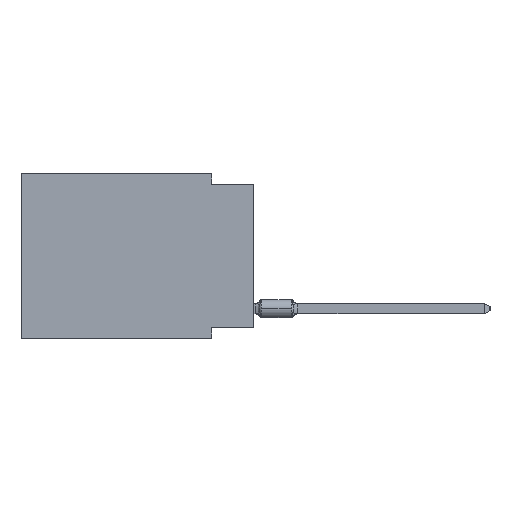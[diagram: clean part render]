
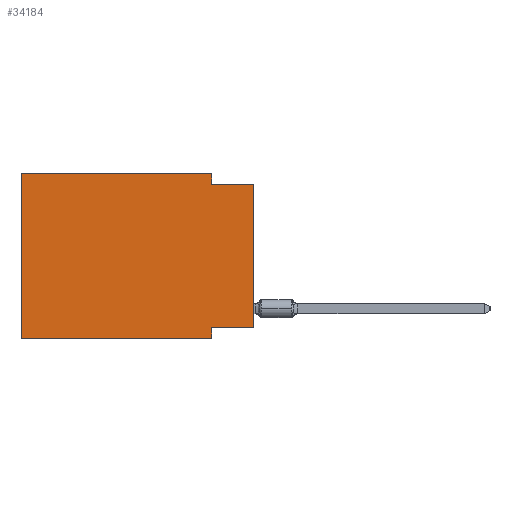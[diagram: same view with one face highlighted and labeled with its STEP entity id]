
A CAD part, left-side view. The second image highlights one B-rep face of the part: STEP entity #34184.
In plain terms, the highlighted planar face has unit normal (-1, 0, 0).
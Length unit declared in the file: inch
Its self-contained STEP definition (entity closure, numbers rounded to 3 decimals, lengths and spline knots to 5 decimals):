
#429 = VECTOR ( 'NONE', #16689, 39.37008 ) ;
#627 = EDGE_CURVE ( 'NONE', #7368, #34009, #24942, .T. ) ;
#677 = VERTEX_POINT ( 'NONE', #8604 ) ;
#1767 = PLANE ( 'NONE',  #8205 ) ;
#2180 = DIRECTION ( 'NONE',  ( 0., 0., 1. ) ) ;
#2861 = DIRECTION ( 'NONE',  ( 0., 0., -1. ) ) ;
#3881 = CARTESIAN_POINT ( 'NONE',  ( 0., 0.55, 0. ) ) ;
#3949 = ORIENTED_EDGE ( 'NONE', *, *, #627, .F. ) ;
#4445 = DIRECTION ( 'NONE',  ( 0., 0., -1. ) ) ;
#4621 = EDGE_LOOP ( 'NONE', ( #34359, #3949, #6401, #26085, #5821, #31547, #30589, #5751 ) ) ;
#4941 = CARTESIAN_POINT ( 'NONE',  ( 0., 0.55, -0.39 ) ) ;
#5213 = VECTOR ( 'NONE', #2861, 39.37008 ) ;
#5252 = VERTEX_POINT ( 'NONE', #3881 ) ;
#5419 = CARTESIAN_POINT ( 'NONE',  ( 0., 0.1, 0. ) ) ;
#5643 = CARTESIAN_POINT ( 'NONE',  ( 0., 0., -0.025 ) ) ;
#5751 = ORIENTED_EDGE ( 'NONE', *, *, #22914, .F. ) ;
#5821 = ORIENTED_EDGE ( 'NONE', *, *, #23498, .F. ) ;
#6401 = ORIENTED_EDGE ( 'NONE', *, *, #6893, .F. ) ;
#6648 = CARTESIAN_POINT ( 'NONE',  ( 0., 0., -0.365 ) ) ;
#6893 = EDGE_CURVE ( 'NONE', #10375, #7368, #22031, .T. ) ;
#7368 = VERTEX_POINT ( 'NONE', #21632 ) ;
#7460 = LINE ( 'NONE', #28712, #13369 ) ;
#7927 = VECTOR ( 'NONE', #4445, 39.37008 ) ;
#8205 = AXIS2_PLACEMENT_3D ( 'NONE', #25989, #28633, #14948 ) ;
#8383 = LINE ( 'NONE', #21924, #10924 ) ;
#8421 = CARTESIAN_POINT ( 'NONE',  ( 0., 0., -0.025 ) ) ;
#8604 = CARTESIAN_POINT ( 'NONE',  ( 0., 0.1, -0.365 ) ) ;
#9453 = LINE ( 'NONE', #6648, #29624 ) ;
#9874 = DIRECTION ( 'NONE',  ( 0., 0., 1. ) ) ;
#10375 = VERTEX_POINT ( 'NONE', #5419 ) ;
#10924 = VECTOR ( 'NONE', #32270, 39.37008 ) ;
#11708 = EDGE_CURVE ( 'NONE', #5252, #10375, #8383, .T. ) ;
#13369 = VECTOR ( 'NONE', #2180, 39.37008 ) ;
#14948 = DIRECTION ( 'NONE',  ( 0., 0., -1. ) ) ;
#15497 = LINE ( 'NONE', #25687, #28084 ) ;
#15819 = VECTOR ( 'NONE', #31308, 39.37008 ) ;
#16689 = DIRECTION ( 'NONE',  ( 0., -1., 0. ) ) ;
#16751 = CARTESIAN_POINT ( 'NONE',  ( 0., 0.1, 0. ) ) ;
#20670 = EDGE_CURVE ( 'NONE', #31798, #34009, #15497, .T. ) ;
#21632 = CARTESIAN_POINT ( 'NONE',  ( 0., 0.1, -0.025 ) ) ;
#21763 = CARTESIAN_POINT ( 'NONE',  ( 0., 0., -0.365 ) ) ;
#21790 = EDGE_CURVE ( 'NONE', #21901, #29143, #34292, .T. ) ;
#21901 = VERTEX_POINT ( 'NONE', #33774 ) ;
#21924 = CARTESIAN_POINT ( 'NONE',  ( 0., 0.55, 0. ) ) ;
#22031 = LINE ( 'NONE', #16751, #5213 ) ;
#22914 = EDGE_CURVE ( 'NONE', #31798, #677, #9453, .T. ) ;
#23498 = EDGE_CURVE ( 'NONE', #21901, #5252, #7460, .T. ) ;
#24942 = LINE ( 'NONE', #8421, #429 ) ;
#25664 = CARTESIAN_POINT ( 'NONE',  ( 0., 0.1, -0.39 ) ) ;
#25687 = CARTESIAN_POINT ( 'NONE',  ( 0., 0., 0. ) ) ;
#25989 = CARTESIAN_POINT ( 'NONE',  ( 0., 0.55, 0. ) ) ;
#26085 = ORIENTED_EDGE ( 'NONE', *, *, #11708, .F. ) ;
#26813 = FACE_OUTER_BOUND ( 'NONE', #4621, .T. ) ;
#27736 = DIRECTION ( 'NONE',  ( 0., 1., 0. ) ) ;
#28084 = VECTOR ( 'NONE', #9874, 39.37008 ) ;
#28507 = CARTESIAN_POINT ( 'NONE',  ( 0., 0.1, -0.39 ) ) ;
#28633 = DIRECTION ( 'NONE',  ( 1., 0., 0. ) ) ;
#28712 = CARTESIAN_POINT ( 'NONE',  ( 0., 0.55, 0. ) ) ;
#28848 = EDGE_CURVE ( 'NONE', #677, #29143, #31147, .T. ) ;
#29143 = VERTEX_POINT ( 'NONE', #25664 ) ;
#29624 = VECTOR ( 'NONE', #27736, 39.37008 ) ;
#30589 = ORIENTED_EDGE ( 'NONE', *, *, #28848, .F. ) ;
#31147 = LINE ( 'NONE', #28507, #7927 ) ;
#31308 = DIRECTION ( 'NONE',  ( 0., -1., 0. ) ) ;
#31547 = ORIENTED_EDGE ( 'NONE', *, *, #21790, .T. ) ;
#31798 = VERTEX_POINT ( 'NONE', #21763 ) ;
#32270 = DIRECTION ( 'NONE',  ( 0., -1., 0. ) ) ;
#33774 = CARTESIAN_POINT ( 'NONE',  ( 0., 0.55, -0.39 ) ) ;
#34009 = VERTEX_POINT ( 'NONE', #5643 ) ;
#34184 = ADVANCED_FACE ( 'NONE', ( #26813 ), #1767, .F. ) ;
#34292 = LINE ( 'NONE', #4941, #15819 ) ;
#34359 = ORIENTED_EDGE ( 'NONE', *, *, #20670, .T. ) ;
